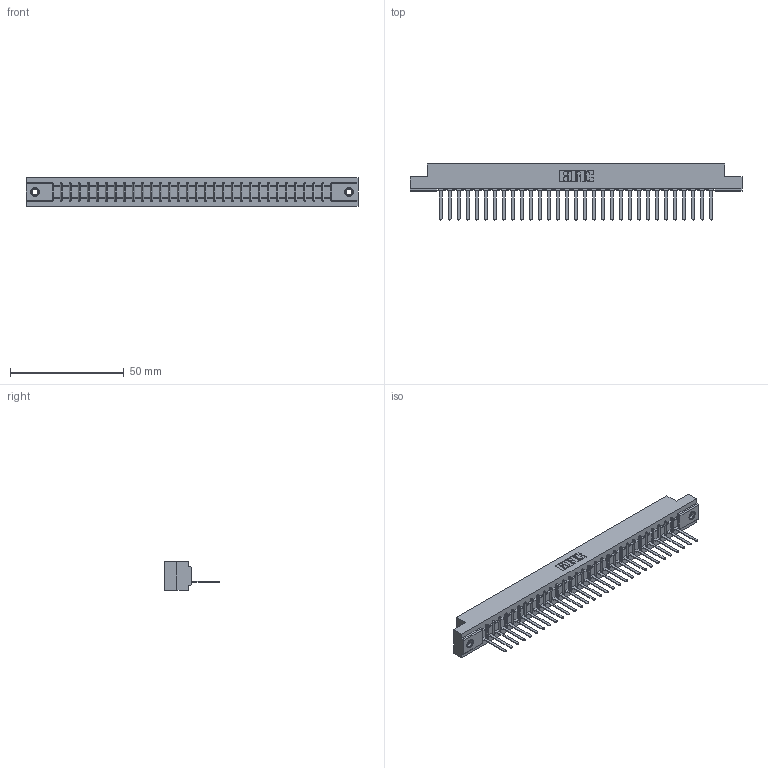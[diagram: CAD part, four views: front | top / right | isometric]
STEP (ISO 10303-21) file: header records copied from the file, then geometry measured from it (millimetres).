
FILE_DESCRIPTION (( 'STEP AP203' ), '1' );
FILE_NAME ('307-031-441-107.STEP', '2020-09-28T14:12:56', ( '' ), ( '' ), 'SwSTEP 2.0', 'SolidWorks 2020', '' );
FILE_SCHEMA (( 'CONFIG_CONTROL_DESIGN' ));
Length unit declared in the file: inch
Products named in the file (4): 307-031-441-107; 307-290-002_541; 345-250-001_345-250-005-103; 307 Part_.156 Dia Mounting Holes
Assembly tree (34 placements, depth 2):
  307-031-441-107
    307 Part_.156 Dia Mounting Holes
    307-290-002_541  x31
    345-250-001_345-250-005-103  x2
Bounding box: 145.85 x 24.59 x 12.7 mm (x, y, z)
Volume: 15599.4 mm3; surface area: 19968.8 mm2
Topology: 34 solids, 34 shells, 2504 faces, 7651 edges, 5006 vertices
Faces by surface type: plane 1497, cylinder 927, sphere 64, cone 12, torus 4
Entity records: 29835 total; most frequent: CARTESIAN_POINT 5011, ORIENTED_EDGE 4994, DIRECTION 4883, EDGE_CURVE 2497, LINE 1907, VECTOR 1907, VERTEX_POINT 1616, AXIS2_PLACEMENT_3D 1488
